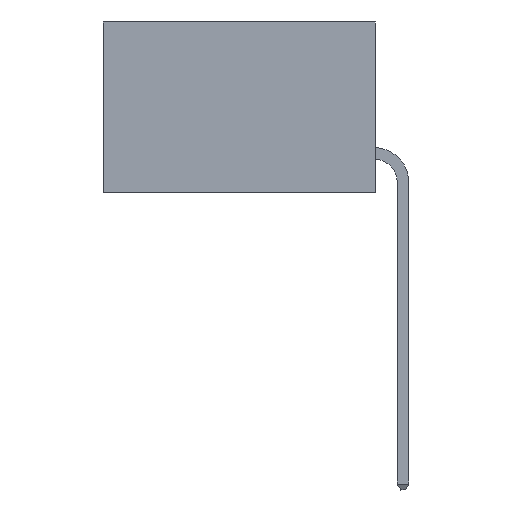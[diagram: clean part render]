
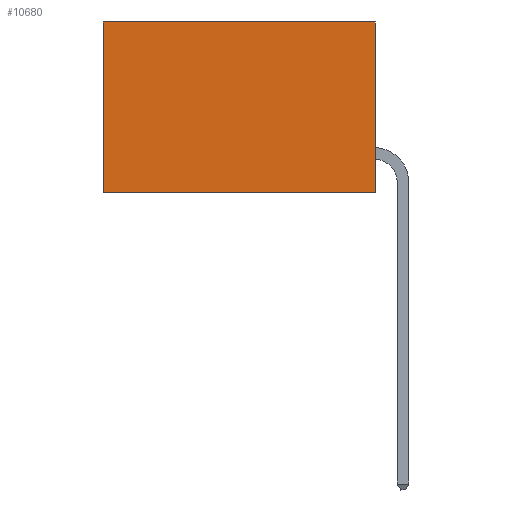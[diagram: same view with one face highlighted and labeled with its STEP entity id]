
A CAD part, left-side view. The second image highlights one B-rep face of the part: STEP entity #10680.
In plain terms, the highlighted planar face has unit normal (-1, 0, 0).
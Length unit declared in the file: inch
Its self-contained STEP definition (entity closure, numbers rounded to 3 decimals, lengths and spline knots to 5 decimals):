
#99 = ORIENTED_EDGE ( 'NONE', *, *, #1500, .F. ) ;
#217 = VERTEX_POINT ( 'NONE', #3946 ) ;
#230 = LINE ( 'NONE', #10860, #6108 ) ;
#1447 = ORIENTED_EDGE ( 'NONE', *, *, #3253, .T. ) ;
#1500 = EDGE_CURVE ( 'NONE', #10584, #11869, #12294, .T. ) ;
#1617 = DIRECTION ( 'NONE',  ( 0., 1., 0. ) ) ;
#2390 = DIRECTION ( 'NONE',  ( 1., 0., 0. ) ) ;
#2402 = LINE ( 'NONE', #8241, #13872 ) ;
#2779 = ORIENTED_EDGE ( 'NONE', *, *, #6577, .F. ) ;
#2963 = VECTOR ( 'NONE', #12453, 39.37008 ) ;
#3253 = EDGE_CURVE ( 'NONE', #10584, #14292, #2402, .T. ) ;
#3375 = VECTOR ( 'NONE', #7753, 39.37008 ) ;
#3946 = CARTESIAN_POINT ( 'NONE',  ( 0.277, 0.59, -0.37 ) ) ;
#4273 = EDGE_CURVE ( 'NONE', #14292, #217, #9443, .T. ) ;
#5149 = CARTESIAN_POINT ( 'NONE',  ( 0.277, 0.59, -0.37 ) ) ;
#5947 = CARTESIAN_POINT ( 'NONE',  ( 0.277, 0., -0.37 ) ) ;
#5970 = EDGE_LOOP ( 'NONE', ( #9335, #2779, #99, #1447 ) ) ;
#6038 = CARTESIAN_POINT ( 'NONE',  ( 0.277, 0., -0.37 ) ) ;
#6108 = VECTOR ( 'NONE', #7696, 39.37008 ) ;
#6577 = EDGE_CURVE ( 'NONE', #11869, #217, #230, .T. ) ;
#7683 = AXIS2_PLACEMENT_3D ( 'NONE', #6038, #2390, #10413 ) ;
#7696 = DIRECTION ( 'NONE',  ( 0., 1., 0. ) ) ;
#7753 = DIRECTION ( 'NONE',  ( 0., 0., -1. ) ) ;
#8241 = CARTESIAN_POINT ( 'NONE',  ( 0.277, 0., 0. ) ) ;
#9335 = ORIENTED_EDGE ( 'NONE', *, *, #4273, .T. ) ;
#9443 = LINE ( 'NONE', #5149, #2963 ) ;
#10068 = CARTESIAN_POINT ( 'NONE',  ( 0.277, 0., -0.37 ) ) ;
#10413 = DIRECTION ( 'NONE',  ( 0., 0., -1. ) ) ;
#10584 = VERTEX_POINT ( 'NONE', #14399 ) ;
#10680 = ADVANCED_FACE ( 'NONE', ( #12477 ), #11424, .F. ) ;
#10860 = CARTESIAN_POINT ( 'NONE',  ( 0.277, 0., -0.37 ) ) ;
#11424 = PLANE ( 'NONE',  #7683 ) ;
#11869 = VERTEX_POINT ( 'NONE', #10068 ) ;
#12102 = CARTESIAN_POINT ( 'NONE',  ( 0.277, 0.59, 0. ) ) ;
#12294 = LINE ( 'NONE', #5947, #3375 ) ;
#12453 = DIRECTION ( 'NONE',  ( 0., 0., -1. ) ) ;
#12477 = FACE_OUTER_BOUND ( 'NONE', #5970, .T. ) ;
#13872 = VECTOR ( 'NONE', #1617, 39.37008 ) ;
#14292 = VERTEX_POINT ( 'NONE', #12102 ) ;
#14399 = CARTESIAN_POINT ( 'NONE',  ( 0.277, 0., 0. ) ) ;
